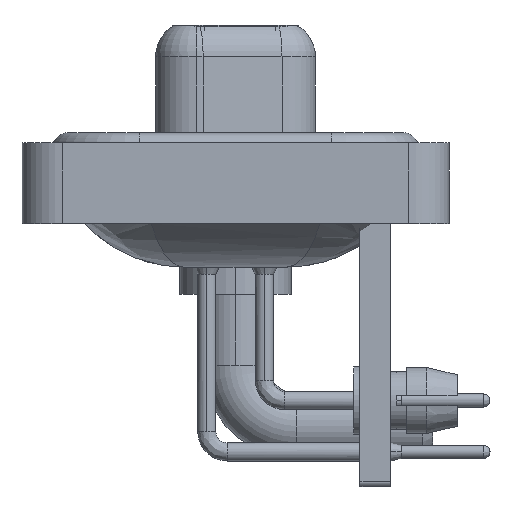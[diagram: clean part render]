
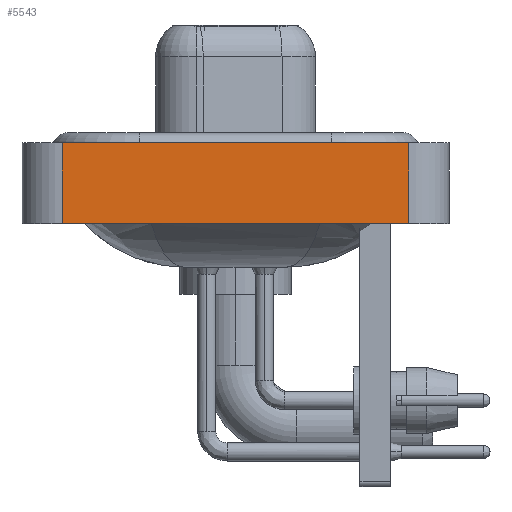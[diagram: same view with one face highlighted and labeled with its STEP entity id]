
A CAD part, left-side view. The second image highlights one B-rep face of the part: STEP entity #5543.
In plain terms, the highlighted planar face has unit normal (-1, 0, 0).
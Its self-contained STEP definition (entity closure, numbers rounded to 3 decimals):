
#118 = CARTESIAN_POINT ( 'NONE',  ( -7.35, -8.55, -3.6 ) ) ;
#567 = CARTESIAN_POINT ( 'NONE',  ( -7.35, 8.55, 0.4 ) ) ;
#706 = VERTEX_POINT ( 'NONE', #25604 ) ;
#1240 = VECTOR ( 'NONE', #12991, 1000. ) ;
#2574 = DIRECTION ( 'NONE',  ( -1., 0., 0. ) ) ;
#2603 = EDGE_CURVE ( 'NONE', #28300, #26626, #22562, .T. ) ;
#5021 = DIRECTION ( 'NONE',  ( 0., -1., 0. ) ) ;
#5543 = ADVANCED_FACE ( 'NONE', ( #24481 ), #22433, .T. ) ;
#6240 = LINE ( 'NONE', #15133, #9270 ) ;
#6380 = DIRECTION ( 'NONE',  ( 0., 0., 1. ) ) ;
#6412 = VERTEX_POINT ( 'NONE', #567 ) ;
#7654 = VECTOR ( 'NONE', #22986, 1000. ) ;
#8716 = ORIENTED_EDGE ( 'NONE', *, *, #22634, .T. ) ;
#9270 = VECTOR ( 'NONE', #6380, 1000. ) ;
#12991 = DIRECTION ( 'NONE',  ( 0., 0., 1. ) ) ;
#13083 = ORIENTED_EDGE ( 'NONE', *, *, #24807, .F. ) ;
#14722 = EDGE_CURVE ( 'NONE', #6412, #706, #15832, .T. ) ;
#14786 = ORIENTED_EDGE ( 'NONE', *, *, #14722, .F. ) ;
#15133 = CARTESIAN_POINT ( 'NONE',  ( -7.35, 8.55, -3.6 ) ) ;
#15832 = LINE ( 'NONE', #24601, #25332 ) ;
#17525 = LINE ( 'NONE', #28777, #1240 ) ;
#18677 = CARTESIAN_POINT ( 'NONE',  ( -7.35, 8.55, -3.6 ) ) ;
#21780 = CARTESIAN_POINT ( 'NONE',  ( -7.35, -8.55, -3.6 ) ) ;
#22268 = ORIENTED_EDGE ( 'NONE', *, *, #2603, .T. ) ;
#22433 = PLANE ( 'NONE',  #28648 ) ;
#22562 = LINE ( 'NONE', #27230, #7654 ) ;
#22634 = EDGE_CURVE ( 'NONE', #26626, #706, #17525, .T. ) ;
#22986 = DIRECTION ( 'NONE',  ( 0., -1., 0. ) ) ;
#24481 = FACE_OUTER_BOUND ( 'NONE', #27280, .T. ) ;
#24601 = CARTESIAN_POINT ( 'NONE',  ( -7.35, -8.55, 0.4 ) ) ;
#24807 = EDGE_CURVE ( 'NONE', #28300, #6412, #6240, .T. ) ;
#25332 = VECTOR ( 'NONE', #5021, 1000. ) ;
#25604 = CARTESIAN_POINT ( 'NONE',  ( -7.35, -8.55, 0.4 ) ) ;
#26626 = VERTEX_POINT ( 'NONE', #21780 ) ;
#26955 = DIRECTION ( 'NONE',  ( 0., 0., 1. ) ) ;
#27230 = CARTESIAN_POINT ( 'NONE',  ( -7.35, -8.55, -3.6 ) ) ;
#27280 = EDGE_LOOP ( 'NONE', ( #8716, #14786, #13083, #22268 ) ) ;
#28300 = VERTEX_POINT ( 'NONE', #18677 ) ;
#28648 = AXIS2_PLACEMENT_3D ( 'NONE', #118, #2574, #26955 ) ;
#28777 = CARTESIAN_POINT ( 'NONE',  ( -7.35, -8.55, -3.6 ) ) ;
